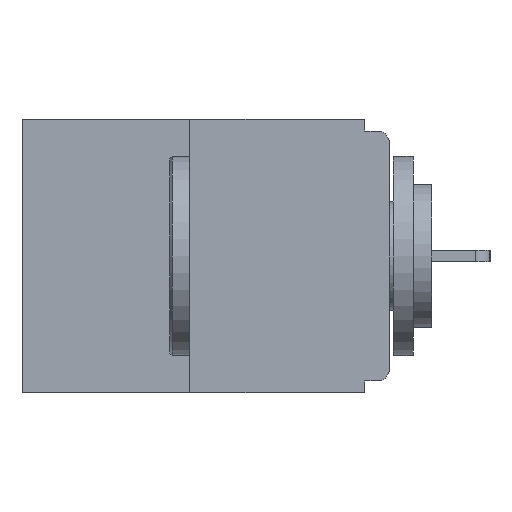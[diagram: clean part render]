
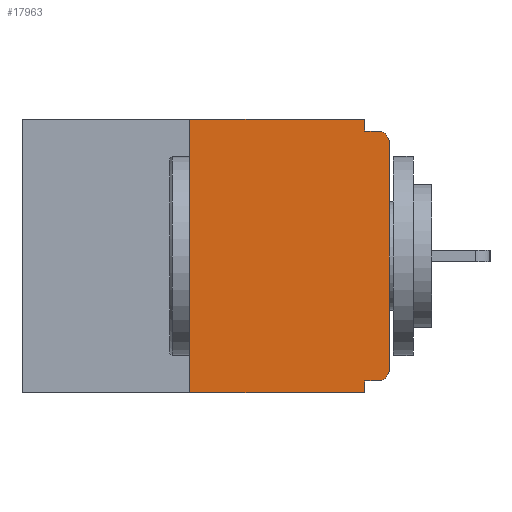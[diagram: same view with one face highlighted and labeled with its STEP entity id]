
A CAD part, left-side view. The second image highlights one B-rep face of the part: STEP entity #17963.
In plain terms, the highlighted planar face has unit normal (-1, 0, 0).
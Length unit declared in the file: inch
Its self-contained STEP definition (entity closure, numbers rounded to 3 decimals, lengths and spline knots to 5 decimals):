
#21 = CARTESIAN_POINT ( 'NONE',  ( 0., 0., -0.03 ) ) ;
#187 = DIRECTION ( 'NONE',  ( -1., 0., 0. ) ) ;
#214 = CARTESIAN_POINT ( 'NONE',  ( 0., 0., 0. ) ) ;
#1826 = EDGE_CURVE ( 'NONE', #10025, #15491, #5006, .T. ) ;
#1968 = CIRCLE ( 'NONE', #18709, 0.015 ) ;
#2005 = VECTOR ( 'NONE', #9944, 39.37008 ) ;
#2036 = LINE ( 'NONE', #20192, #13700 ) ;
#2352 = CARTESIAN_POINT ( 'NONE',  ( 0., 0.015, -0.015 ) ) ;
#2573 = CIRCLE ( 'NONE', #20459, 0.015 ) ;
#3055 = CARTESIAN_POINT ( 'NONE',  ( 0., 0.015, -0.328 ) ) ;
#3078 = DIRECTION ( 'NONE',  ( 0., -1., 0. ) ) ;
#3188 = DIRECTION ( 'NONE',  ( 1., 0., 0. ) ) ;
#3526 = VERTEX_POINT ( 'NONE', #21 ) ;
#3633 = ORIENTED_EDGE ( 'NONE', *, *, #7006, .F. ) ;
#4413 = CARTESIAN_POINT ( 'NONE',  ( 0., 0., -0.328 ) ) ;
#4746 = AXIS2_PLACEMENT_3D ( 'NONE', #12201, #3188, #19654 ) ;
#4789 = LINE ( 'NONE', #12205, #18025 ) ;
#5006 = LINE ( 'NONE', #10126, #21872 ) ;
#5012 = EDGE_CURVE ( 'NONE', #14157, #6248, #17809, .T. ) ;
#5162 = DIRECTION ( 'NONE',  ( 0., 0., -1. ) ) ;
#5891 = ORIENTED_EDGE ( 'NONE', *, *, #8699, .F. ) ;
#6248 = VERTEX_POINT ( 'NONE', #2352 ) ;
#6354 = CARTESIAN_POINT ( 'NONE',  ( 0., 0., -0.313 ) ) ;
#6991 = DIRECTION ( 'NONE',  ( -1., 0., 0. ) ) ;
#7006 = EDGE_CURVE ( 'NONE', #22895, #21657, #11359, .T. ) ;
#7676 = LINE ( 'NONE', #4413, #10697 ) ;
#7870 = CARTESIAN_POINT ( 'NONE',  ( 0., 0.46, -0.343 ) ) ;
#8473 = EDGE_CURVE ( 'NONE', #3526, #6248, #2573, .T. ) ;
#8699 = EDGE_CURVE ( 'NONE', #21783, #10025, #7676, .T. ) ;
#9046 = CARTESIAN_POINT ( 'NONE',  ( 0., 0.015, -0.03 ) ) ;
#9460 = ORIENTED_EDGE ( 'NONE', *, *, #13166, .F. ) ;
#9944 = DIRECTION ( 'NONE',  ( 0., 0., 1. ) ) ;
#10025 = VERTEX_POINT ( 'NONE', #19630 ) ;
#10126 = CARTESIAN_POINT ( 'NONE',  ( 0., 0.031, -0.343 ) ) ;
#10340 = DIRECTION ( 'NONE',  ( 0., -1., 0. ) ) ;
#10697 = VECTOR ( 'NONE', #15376, 39.37008 ) ;
#11177 = CARTESIAN_POINT ( 'NONE',  ( 0., 0.031, -0.343 ) ) ;
#11359 = LINE ( 'NONE', #16361, #16407 ) ;
#11630 = ORIENTED_EDGE ( 'NONE', *, *, #5012, .F. ) ;
#12201 = CARTESIAN_POINT ( 'NONE',  ( 0., 0.46, 0. ) ) ;
#12205 = CARTESIAN_POINT ( 'NONE',  ( 0., 0.46, 0. ) ) ;
#12211 = VECTOR ( 'NONE', #21310, 39.37008 ) ;
#13166 = EDGE_CURVE ( 'NONE', #21657, #21496, #4789, .T. ) ;
#13649 = ORIENTED_EDGE ( 'NONE', *, *, #8473, .T. ) ;
#13700 = VECTOR ( 'NONE', #22043, 39.37008 ) ;
#13926 = ORIENTED_EDGE ( 'NONE', *, *, #1826, .F. ) ;
#14004 = EDGE_LOOP ( 'NONE', ( #9460, #3633, #19358, #13926, #5891, #23123, #16751, #13649, #11630, #15667 ) ) ;
#14040 = FACE_OUTER_BOUND ( 'NONE', #14004, .T. ) ;
#14157 = VERTEX_POINT ( 'NONE', #20191 ) ;
#15376 = DIRECTION ( 'NONE',  ( 0., 1., 0. ) ) ;
#15491 = VERTEX_POINT ( 'NONE', #11177 ) ;
#15625 = CARTESIAN_POINT ( 'NONE',  ( 0., 0., -0.015 ) ) ;
#15667 = ORIENTED_EDGE ( 'NONE', *, *, #15876, .F. ) ;
#15876 = EDGE_CURVE ( 'NONE', #21496, #14157, #2036, .T. ) ;
#16361 = CARTESIAN_POINT ( 'NONE',  ( 0., 0.25, 0. ) ) ;
#16407 = VECTOR ( 'NONE', #20270, 39.37008 ) ;
#16751 = ORIENTED_EDGE ( 'NONE', *, *, #16857, .T. ) ;
#16857 = EDGE_CURVE ( 'NONE', #21777, #3526, #16912, .T. ) ;
#16912 = LINE ( 'NONE', #214, #2005 ) ;
#17475 = DIRECTION ( 'NONE',  ( 0., 0., -1. ) ) ;
#17763 = CARTESIAN_POINT ( 'NONE',  ( 0., 0.25, -0.343 ) ) ;
#17809 = LINE ( 'NONE', #15625, #21622 ) ;
#17939 = PLANE ( 'NONE',  #4746 ) ;
#17963 = ADVANCED_FACE ( 'NONE', ( #14040 ), #17939, .F. ) ;
#18025 = VECTOR ( 'NONE', #3078, 39.37008 ) ;
#18305 = CARTESIAN_POINT ( 'NONE',  ( 0., 0.031, 0. ) ) ;
#18709 = AXIS2_PLACEMENT_3D ( 'NONE', #21658, #6991, #5162 ) ;
#19358 = ORIENTED_EDGE ( 'NONE', *, *, #19805, .T. ) ;
#19630 = CARTESIAN_POINT ( 'NONE',  ( 0., 0.031, -0.328 ) ) ;
#19654 = DIRECTION ( 'NONE',  ( 0., 0., -1. ) ) ;
#19805 = EDGE_CURVE ( 'NONE', #22895, #15491, #20815, .T. ) ;
#20191 = CARTESIAN_POINT ( 'NONE',  ( 0., 0.031, -0.015 ) ) ;
#20192 = CARTESIAN_POINT ( 'NONE',  ( 0., 0.031, 0. ) ) ;
#20270 = DIRECTION ( 'NONE',  ( 0., 0., 1. ) ) ;
#20369 = EDGE_CURVE ( 'NONE', #21783, #21777, #1968, .T. ) ;
#20418 = DIRECTION ( 'NONE',  ( 0., 0., -1. ) ) ;
#20459 = AXIS2_PLACEMENT_3D ( 'NONE', #9046, #187, #20418 ) ;
#20815 = LINE ( 'NONE', #7870, #12211 ) ;
#21310 = DIRECTION ( 'NONE',  ( 0., -1., 0. ) ) ;
#21496 = VERTEX_POINT ( 'NONE', #18305 ) ;
#21622 = VECTOR ( 'NONE', #10340, 39.37008 ) ;
#21657 = VERTEX_POINT ( 'NONE', #23321 ) ;
#21658 = CARTESIAN_POINT ( 'NONE',  ( 0., 0.015, -0.313 ) ) ;
#21777 = VERTEX_POINT ( 'NONE', #6354 ) ;
#21783 = VERTEX_POINT ( 'NONE', #3055 ) ;
#21872 = VECTOR ( 'NONE', #17475, 39.37008 ) ;
#22043 = DIRECTION ( 'NONE',  ( 0., 0., -1. ) ) ;
#22895 = VERTEX_POINT ( 'NONE', #17763 ) ;
#23123 = ORIENTED_EDGE ( 'NONE', *, *, #20369, .T. ) ;
#23321 = CARTESIAN_POINT ( 'NONE',  ( 0., 0.25, 0. ) ) ;
